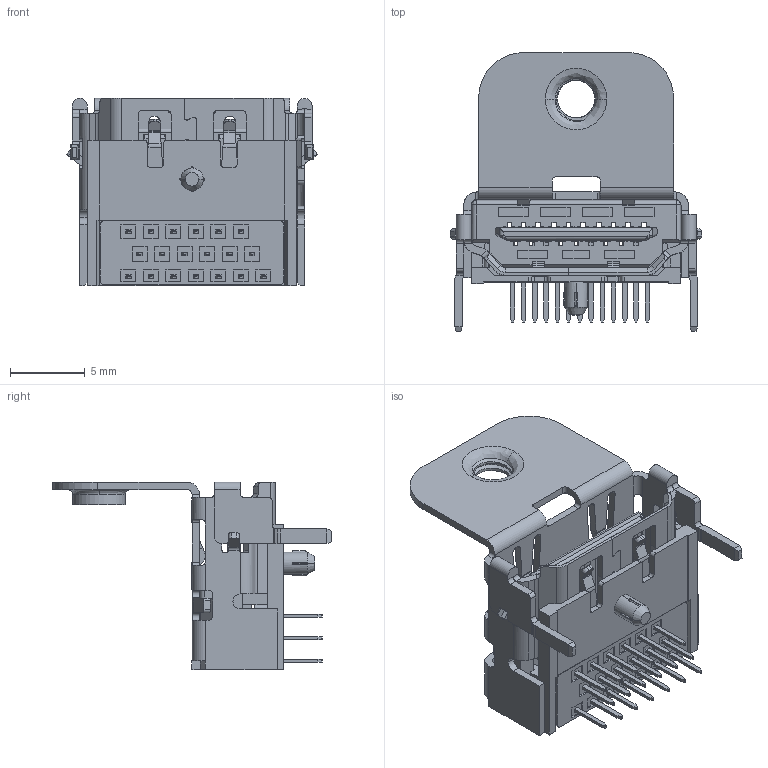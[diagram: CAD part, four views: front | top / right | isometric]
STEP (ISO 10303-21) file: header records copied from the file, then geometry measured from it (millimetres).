
FILE_DESCRIPTION (( 'STEP AP214' ), '1' );
FILE_NAME ('694B119-127-711.STEP', '2021-01-13T14:16:11', ( '' ), ( '' ), 'SwSTEP 2.0', 'SolidWorks 2020', '' );
FILE_SCHEMA (( 'AUTOMOTIVE_DESIGN' ));
Length unit declared in the file: millimetre
Products named in the file (23): Contact 6 694B119-X27-711; Contact 14 694B119-X27-711; Contact 8 694B119-X27-711; Contact 7 694B119-X27-711; Contact 11 694B119-X27-711; Contact 4 694B119-X27-711; Contact 16 694B119-X27-711; Contact 17 694B119-X27-711; Contact 5 694B119-X27-711; Contact 1 694B119-X27-711; Contact 18 694B119-X27-711; Contact 12 694B119-X27-711; Contact 19 694B119-X27-711; Contact 10 694B119-X27-711; Contact 15 694B119-X27-711; Shell 694B119-X27-711; Contact 13 694B119-X27-711; Contact 2 694B119-X27-711; Insulator 694B119-X27-711; Insulator2 694B119-X27-711; Contact 9 694B119-X27-711; 694B119-127-711; Contact 3 694B119-X27-711
Assembly tree (22 placements, depth 2):
  694B119-127-711
    Insulator 694B119-X27-711
    Contact 2 694B119-X27-711
    Contact 4 694B119-X27-711
    Contact 6 694B119-X27-711
    Contact 8 694B119-X27-711
    Contact 10 694B119-X27-711
    Contact 12 694B119-X27-711
    Contact 14 694B119-X27-711
    Contact 16 694B119-X27-711
    Contact 18 694B119-X27-711
    Contact 1 694B119-X27-711
    Contact 3 694B119-X27-711
    Contact 5 694B119-X27-711
    Contact 7 694B119-X27-711
    Contact 9 694B119-X27-711
    Contact 11 694B119-X27-711
    Contact 13 694B119-X27-711
    Contact 15 694B119-X27-711
    Contact 17 694B119-X27-711
    Contact 19 694B119-X27-711
    Insulator2 694B119-X27-711
    Shell 694B119-X27-711
Bounding box: 16.75 x 18.6 x 12.5 mm (x, y, z)
Volume: 603.1 mm3; surface area: 2597 mm2
Topology: 22 solids, 22 shells, 2042 faces, 5757 edges, 3727 vertices
Faces by surface type: plane 1664, cylinder 326, bspline 48, cone 4
Entity records: 68666 total; most frequent: CARTESIAN_POINT 15183, ORIENTED_EDGE 11512, DIRECTION 10022, EDGE_CURVE 5756, LINE 4928, VECTOR 4928, VERTEX_POINT 3728, AXIS2_PLACEMENT_3D 2547
